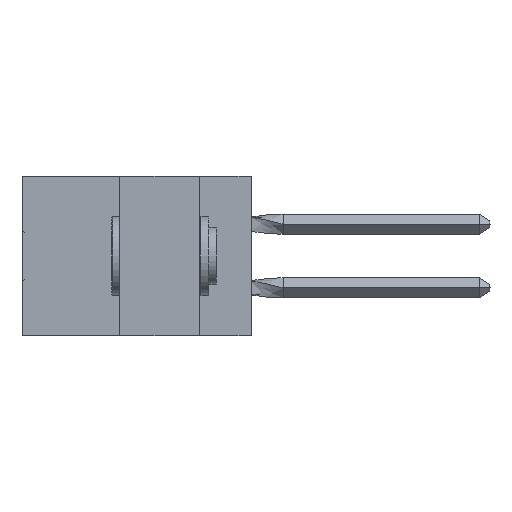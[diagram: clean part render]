
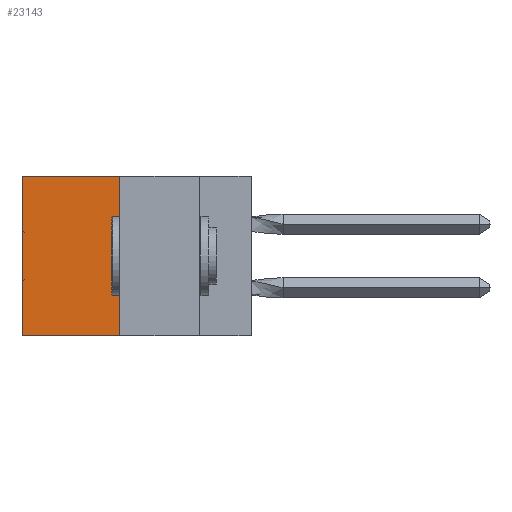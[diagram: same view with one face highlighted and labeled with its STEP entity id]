
A CAD part, left-side view. The second image highlights one B-rep face of the part: STEP entity #23143.
In plain terms, the highlighted planar face has unit normal (-1, 0, 0).
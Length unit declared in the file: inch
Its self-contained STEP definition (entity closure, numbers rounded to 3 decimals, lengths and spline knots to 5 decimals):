
#2355 = VECTOR ( 'NONE', #23416, 39.37008 ) ;
#2518 = LINE ( 'NONE', #15413, #48894 ) ;
#4387 = EDGE_CURVE ( 'NONE', #45660, #49028, #2518, .T. ) ;
#6309 = CARTESIAN_POINT ( 'NONE',  ( 0.305, 0.413, -0.5 ) ) ;
#6680 = DIRECTION ( 'NONE',  ( 1., 0., 0. ) ) ;
#8578 = CARTESIAN_POINT ( 'NONE',  ( 0.305, 0.413, -0.5 ) ) ;
#10470 = CARTESIAN_POINT ( 'NONE',  ( 0.305, 0.413, 0. ) ) ;
#11123 = LINE ( 'NONE', #19311, #37715 ) ;
#11568 = DIRECTION ( 'NONE',  ( 0., 1., 0. ) ) ;
#12566 = AXIS2_PLACEMENT_3D ( 'NONE', #34647, #6680, #30482 ) ;
#12587 = LINE ( 'NONE', #6309, #41108 ) ;
#15413 = CARTESIAN_POINT ( 'NONE',  ( 0.305, 0.413, -0.5 ) ) ;
#15821 = VERTEX_POINT ( 'NONE', #50950 ) ;
#19311 = CARTESIAN_POINT ( 'NONE',  ( 0.305, 0.413, 0. ) ) ;
#19664 = ORIENTED_EDGE ( 'NONE', *, *, #25594, .T. ) ;
#22078 = ORIENTED_EDGE ( 'NONE', *, *, #28919, .T. ) ;
#23033 = FACE_OUTER_BOUND ( 'NONE', #26751, .T. ) ;
#23034 = PLANE ( 'NONE',  #12566 ) ;
#23143 = ADVANCED_FACE ( 'NONE', ( #23033 ), #23034, .F. ) ;
#23416 = DIRECTION ( 'NONE',  ( 0., 0., -1. ) ) ;
#25594 = EDGE_CURVE ( 'NONE', #50675, #15821, #37610, .T. ) ;
#26751 = EDGE_LOOP ( 'NONE', ( #19664, #38318, #38264, #22078 ) ) ;
#28919 = EDGE_CURVE ( 'NONE', #45660, #50675, #11123, .T. ) ;
#29572 = DIRECTION ( 'NONE',  ( 0., 1., 0. ) ) ;
#30482 = DIRECTION ( 'NONE',  ( 0., 0., -1. ) ) ;
#31814 = CARTESIAN_POINT ( 'NONE',  ( 0.305, 0.72, 0. ) ) ;
#34647 = CARTESIAN_POINT ( 'NONE',  ( 0.305, 0.413, -0.5 ) ) ;
#35538 = CARTESIAN_POINT ( 'NONE',  ( 0.305, 0.72, -0.5 ) ) ;
#37610 = LINE ( 'NONE', #35538, #2355 ) ;
#37715 = VECTOR ( 'NONE', #11568, 39.37008 ) ;
#38264 = ORIENTED_EDGE ( 'NONE', *, *, #4387, .F. ) ;
#38318 = ORIENTED_EDGE ( 'NONE', *, *, #44300, .F. ) ;
#41108 = VECTOR ( 'NONE', #29572, 39.37008 ) ;
#43296 = DIRECTION ( 'NONE',  ( 0., 0., -1. ) ) ;
#44300 = EDGE_CURVE ( 'NONE', #49028, #15821, #12587, .T. ) ;
#45660 = VERTEX_POINT ( 'NONE', #10470 ) ;
#48894 = VECTOR ( 'NONE', #43296, 39.37008 ) ;
#49028 = VERTEX_POINT ( 'NONE', #8578 ) ;
#50675 = VERTEX_POINT ( 'NONE', #31814 ) ;
#50950 = CARTESIAN_POINT ( 'NONE',  ( 0.305, 0.72, -0.5 ) ) ;
